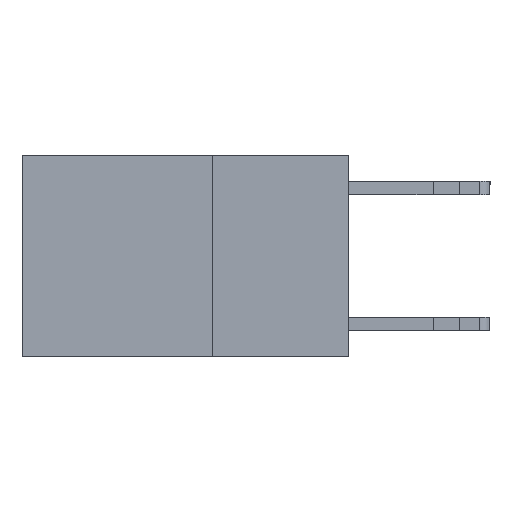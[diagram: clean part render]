
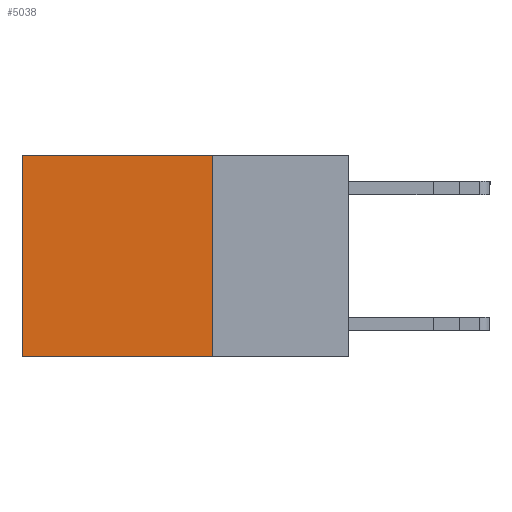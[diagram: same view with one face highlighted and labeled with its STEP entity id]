
A CAD part, left-side view. The second image highlights one B-rep face of the part: STEP entity #5038.
In plain terms, the highlighted planar face has unit normal (-1, 0, 0).
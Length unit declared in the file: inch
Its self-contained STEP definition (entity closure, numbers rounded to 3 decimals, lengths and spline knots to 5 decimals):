
#422 = VECTOR ( 'NONE', #950, 39.37008 ) ;
#881 = FACE_OUTER_BOUND ( 'NONE', #6268, .T. ) ;
#950 = DIRECTION ( 'NONE',  ( 0., 0., -1. ) ) ;
#1452 = DIRECTION ( 'NONE',  ( 0., 1., 0. ) ) ;
#1542 = ORIENTED_EDGE ( 'NONE', *, *, #6651, .T. ) ;
#1701 = VECTOR ( 'NONE', #1452, 39.37008 ) ;
#1708 = VERTEX_POINT ( 'NONE', #10440 ) ;
#1937 = DIRECTION ( 'NONE',  ( 0., 0., -1. ) ) ;
#1964 = ORIENTED_EDGE ( 'NONE', *, *, #9192, .F. ) ;
#2398 = VERTEX_POINT ( 'NONE', #3246 ) ;
#2825 = VECTOR ( 'NONE', #11791, 39.37008 ) ;
#3246 = CARTESIAN_POINT ( 'NONE',  ( 0.2625, 0.25, 0. ) ) ;
#3421 = VERTEX_POINT ( 'NONE', #10561 ) ;
#3437 = LINE ( 'NONE', #11086, #1701 ) ;
#3852 = CARTESIAN_POINT ( 'NONE',  ( 0.2625, 0.25, 0. ) ) ;
#4884 = LINE ( 'NONE', #8855, #2825 ) ;
#4912 = DIRECTION ( 'NONE',  ( 1., 0., 0. ) ) ;
#5038 = ADVANCED_FACE ( 'NONE', ( #881 ), #11871, .F. ) ;
#5785 = ORIENTED_EDGE ( 'NONE', *, *, #9388, .T. ) ;
#6268 = EDGE_LOOP ( 'NONE', ( #5785, #11790, #1964, #1542 ) ) ;
#6651 = EDGE_CURVE ( 'NONE', #2398, #3421, #4884, .T. ) ;
#8855 = CARTESIAN_POINT ( 'NONE',  ( 0.2625, 0.25, 0. ) ) ;
#8876 = CARTESIAN_POINT ( 'NONE',  ( 0.2625, 0.25, 0. ) ) ;
#9192 = EDGE_CURVE ( 'NONE', #2398, #12743, #10827, .T. ) ;
#9388 = EDGE_CURVE ( 'NONE', #3421, #1708, #9449, .T. ) ;
#9399 = EDGE_CURVE ( 'NONE', #12743, #1708, #3437, .T. ) ;
#9449 = LINE ( 'NONE', #10029, #10942 ) ;
#10029 = CARTESIAN_POINT ( 'NONE',  ( 0.2625, 0.6, 0. ) ) ;
#10440 = CARTESIAN_POINT ( 'NONE',  ( 0.2625, 0.6, -0.37 ) ) ;
#10561 = CARTESIAN_POINT ( 'NONE',  ( 0.2625, 0.6, 0. ) ) ;
#10572 = AXIS2_PLACEMENT_3D ( 'NONE', #8876, #4912, #1937 ) ;
#10827 = LINE ( 'NONE', #3852, #422 ) ;
#10942 = VECTOR ( 'NONE', #12184, 39.37008 ) ;
#11086 = CARTESIAN_POINT ( 'NONE',  ( 0.2625, 0.25, -0.37 ) ) ;
#11790 = ORIENTED_EDGE ( 'NONE', *, *, #9399, .F. ) ;
#11791 = DIRECTION ( 'NONE',  ( 0., 1., 0. ) ) ;
#11871 = PLANE ( 'NONE',  #10572 ) ;
#12184 = DIRECTION ( 'NONE',  ( 0., 0., -1. ) ) ;
#12526 = CARTESIAN_POINT ( 'NONE',  ( 0.2625, 0.25, -0.37 ) ) ;
#12743 = VERTEX_POINT ( 'NONE', #12526 ) ;
